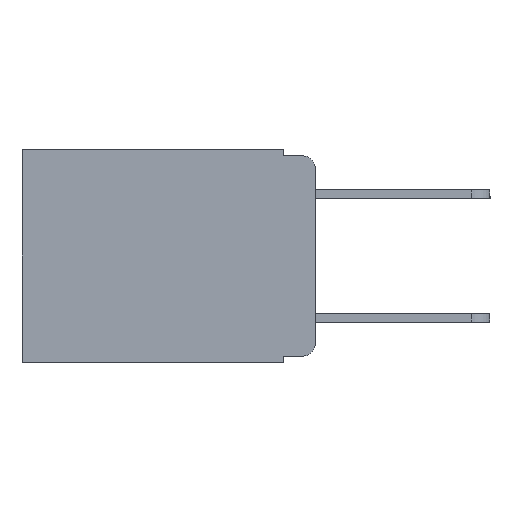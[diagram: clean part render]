
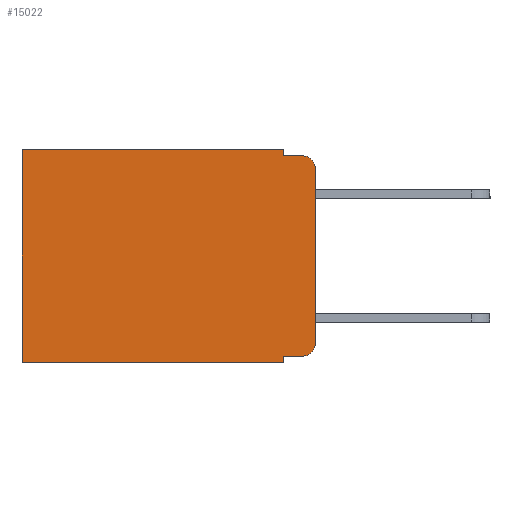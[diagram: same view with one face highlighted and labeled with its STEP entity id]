
A CAD part, left-side view. The second image highlights one B-rep face of the part: STEP entity #15022.
In plain terms, the highlighted planar face has unit normal (-1, 0, 0).
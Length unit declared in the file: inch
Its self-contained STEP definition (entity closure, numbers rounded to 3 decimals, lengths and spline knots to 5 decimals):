
#128 = VERTEX_POINT ( 'NONE', #15039 ) ;
#181 = VECTOR ( 'NONE', #10196, 39.37008 ) ;
#331 = DIRECTION ( 'NONE',  ( 0., 0., -1. ) ) ;
#710 = LINE ( 'NONE', #14024, #14289 ) ;
#959 = ORIENTED_EDGE ( 'NONE', *, *, #10628, .T. ) ;
#1229 = CARTESIAN_POINT ( 'NONE',  ( 0.298, 0.051, -0.333 ) ) ;
#1440 = CARTESIAN_POINT ( 'NONE',  ( 0.298, 0.02, -0.01 ) ) ;
#1841 = LINE ( 'NONE', #16548, #12188 ) ;
#2268 = CARTESIAN_POINT ( 'NONE',  ( 0.298, 0., 0. ) ) ;
#2497 = VECTOR ( 'NONE', #13611, 39.37008 ) ;
#2620 = CARTESIAN_POINT ( 'NONE',  ( 0.298, 0.051, 0. ) ) ;
#3209 = AXIS2_PLACEMENT_3D ( 'NONE', #13045, #4767, #14354 ) ;
#3243 = PLANE ( 'NONE',  #3209 ) ;
#3367 = ORIENTED_EDGE ( 'NONE', *, *, #7714, .T. ) ;
#3376 = CARTESIAN_POINT ( 'NONE',  ( 0.298, 0.051, 0. ) ) ;
#3395 = CARTESIAN_POINT ( 'NONE',  ( 0.298, 0.473, 0. ) ) ;
#3417 = CIRCLE ( 'NONE', #16538, 0.02 ) ;
#3593 = VERTEX_POINT ( 'NONE', #16017 ) ;
#4089 = DIRECTION ( 'NONE',  ( 0., 0., -1. ) ) ;
#4259 = DIRECTION ( 'NONE',  ( 0., -1., 0. ) ) ;
#4650 = ORIENTED_EDGE ( 'NONE', *, *, #5802, .F. ) ;
#4767 = DIRECTION ( 'NONE',  ( 1., 0., 0. ) ) ;
#5080 = ORIENTED_EDGE ( 'NONE', *, *, #10055, .F. ) ;
#5181 = ORIENTED_EDGE ( 'NONE', *, *, #14443, .F. ) ;
#5221 = DIRECTION ( 'NONE',  ( -1., 0., 0. ) ) ;
#5230 = VERTEX_POINT ( 'NONE', #7336 ) ;
#5241 = ORIENTED_EDGE ( 'NONE', *, *, #10668, .F. ) ;
#5252 = CARTESIAN_POINT ( 'NONE',  ( 0.298, 0., -0.03 ) ) ;
#5396 = ORIENTED_EDGE ( 'NONE', *, *, #9712, .T. ) ;
#5674 = DIRECTION ( 'NONE',  ( 0., -1., 0. ) ) ;
#5802 = EDGE_CURVE ( 'NONE', #16112, #7850, #12860, .T. ) ;
#5901 = EDGE_CURVE ( 'NONE', #5230, #128, #710, .T. ) ;
#6397 = ORIENTED_EDGE ( 'NONE', *, *, #6653, .T. ) ;
#6456 = VECTOR ( 'NONE', #17097, 39.37008 ) ;
#6653 = EDGE_CURVE ( 'NONE', #12065, #14345, #7527, .T. ) ;
#6981 = VERTEX_POINT ( 'NONE', #10615 ) ;
#7336 = CARTESIAN_POINT ( 'NONE',  ( 0.298, 0.051, -0.343 ) ) ;
#7504 = CARTESIAN_POINT ( 'NONE',  ( 0.298, 0.02, -0.03 ) ) ;
#7527 = LINE ( 'NONE', #2268, #181 ) ;
#7714 = EDGE_CURVE ( 'NONE', #14345, #128, #13602, .T. ) ;
#7850 = VERTEX_POINT ( 'NONE', #17602 ) ;
#8032 = ORIENTED_EDGE ( 'NONE', *, *, #5901, .F. ) ;
#8666 = CARTESIAN_POINT ( 'NONE',  ( 0.298, 0.051, -0.01 ) ) ;
#8834 = DIRECTION ( 'NONE',  ( 0., 0., -1. ) ) ;
#9618 = LINE ( 'NONE', #17000, #16289 ) ;
#9712 = EDGE_CURVE ( 'NONE', #16112, #10172, #10736, .T. ) ;
#10055 = EDGE_CURVE ( 'NONE', #12065, #12893, #15947, .T. ) ;
#10172 = VERTEX_POINT ( 'NONE', #1440 ) ;
#10196 = DIRECTION ( 'NONE',  ( 0., 1., 0. ) ) ;
#10615 = CARTESIAN_POINT ( 'NONE',  ( 0.298, 0.051, -0.333 ) ) ;
#10628 = EDGE_CURVE ( 'NONE', #6981, #3593, #16551, .T. ) ;
#10668 = EDGE_CURVE ( 'NONE', #12893, #10172, #1841, .T. ) ;
#10736 = CIRCLE ( 'NONE', #10786, 0.02 ) ;
#10786 = AXIS2_PLACEMENT_3D ( 'NONE', #7504, #16878, #8834 ) ;
#12065 = VERTEX_POINT ( 'NONE', #3376 ) ;
#12188 = VECTOR ( 'NONE', #4259, 39.37008 ) ;
#12860 = LINE ( 'NONE', #14392, #6456 ) ;
#12893 = VERTEX_POINT ( 'NONE', #8666 ) ;
#12951 = EDGE_LOOP ( 'NONE', ( #4650, #5396, #5241, #5080, #6397, #3367, #8032, #5181, #959, #14751 ) ) ;
#13045 = CARTESIAN_POINT ( 'NONE',  ( 0.298, 0., 0. ) ) ;
#13445 = CARTESIAN_POINT ( 'NONE',  ( 0.298, 0.02, -0.313 ) ) ;
#13602 = LINE ( 'NONE', #3395, #2497 ) ;
#13611 = DIRECTION ( 'NONE',  ( 0., 0., -1. ) ) ;
#13774 = EDGE_CURVE ( 'NONE', #3593, #7850, #3417, .T. ) ;
#14024 = CARTESIAN_POINT ( 'NONE',  ( 0.298, 0., -0.343 ) ) ;
#14289 = VECTOR ( 'NONE', #16432, 39.37008 ) ;
#14345 = VERTEX_POINT ( 'NONE', #17407 ) ;
#14354 = DIRECTION ( 'NONE',  ( 0., 0., -1. ) ) ;
#14392 = CARTESIAN_POINT ( 'NONE',  ( 0.298, 0., 0. ) ) ;
#14443 = EDGE_CURVE ( 'NONE', #6981, #5230, #9618, .T. ) ;
#14751 = ORIENTED_EDGE ( 'NONE', *, *, #13774, .T. ) ;
#14767 = DIRECTION ( 'NONE',  ( 0., 0., -1. ) ) ;
#15022 = ADVANCED_FACE ( 'NONE', ( #15658 ), #3243, .F. ) ;
#15039 = CARTESIAN_POINT ( 'NONE',  ( 0.298, 0.473, -0.343 ) ) ;
#15658 = FACE_OUTER_BOUND ( 'NONE', #12951, .T. ) ;
#15947 = LINE ( 'NONE', #2620, #16357 ) ;
#16017 = CARTESIAN_POINT ( 'NONE',  ( 0.298, 0.02, -0.333 ) ) ;
#16112 = VERTEX_POINT ( 'NONE', #5252 ) ;
#16124 = VECTOR ( 'NONE', #5674, 39.37008 ) ;
#16289 = VECTOR ( 'NONE', #331, 39.37008 ) ;
#16357 = VECTOR ( 'NONE', #4089, 39.37008 ) ;
#16432 = DIRECTION ( 'NONE',  ( 0., 1., 0. ) ) ;
#16538 = AXIS2_PLACEMENT_3D ( 'NONE', #13445, #5221, #14767 ) ;
#16548 = CARTESIAN_POINT ( 'NONE',  ( 0.298, 0.051, -0.01 ) ) ;
#16551 = LINE ( 'NONE', #1229, #16124 ) ;
#16878 = DIRECTION ( 'NONE',  ( -1., 0., 0. ) ) ;
#17000 = CARTESIAN_POINT ( 'NONE',  ( 0.298, 0.051, 0. ) ) ;
#17097 = DIRECTION ( 'NONE',  ( 0., 0., -1. ) ) ;
#17407 = CARTESIAN_POINT ( 'NONE',  ( 0.298, 0.473, 0. ) ) ;
#17602 = CARTESIAN_POINT ( 'NONE',  ( 0.298, 0., -0.313 ) ) ;
